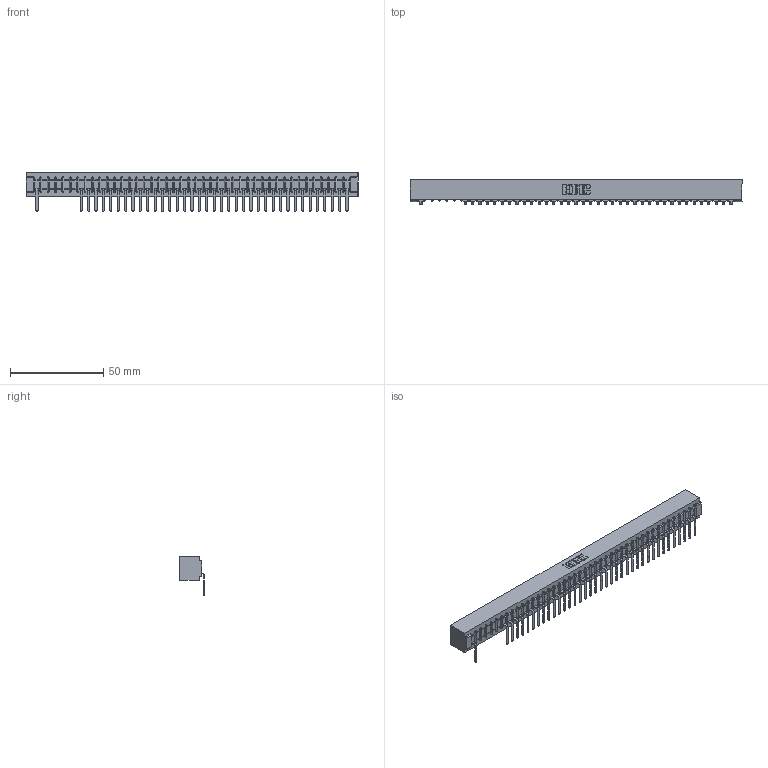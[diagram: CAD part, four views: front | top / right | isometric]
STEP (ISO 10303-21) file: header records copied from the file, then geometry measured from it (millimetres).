
FILE_DESCRIPTION (( 'STEP AP203' ), '1' );
FILE_NAME ('357-043-557-101.STEP', '2018-08-11T10:33:37', ( '' ), ( '' ), 'SwSTEP 2.0', 'SolidWorks 2016', '' );
FILE_SCHEMA (( 'CONFIG_CONTROL_DESIGN' ));
Length unit declared in the file: inch
Products named in the file (3): 307 Part_No Mounting Lugs; 307-290-002_557; 357-043-557-101
Assembly tree (39 placements, depth 2):
  357-043-557-101
    307 Part_No Mounting Lugs
    307-290-002_557  x38
Bounding box: 178.26 x 13.32 x 20.66 mm (x, y, z)
Volume: 19598.8 mm3; surface area: 24754 mm2
Topology: 39 solids, 39 shells, 3218 faces, 9891 edges, 6474 vertices
Faces by surface type: plane 1912, cylinder 1218, sphere 88
Entity records: 37156 total; most frequent: CARTESIAN_POINT 6291, ORIENTED_EDGE 6286, DIRECTION 6105, EDGE_CURVE 3143, LINE 2409, VECTOR 2409, VERTEX_POINT 2034, AXIS2_PLACEMENT_3D 1848
